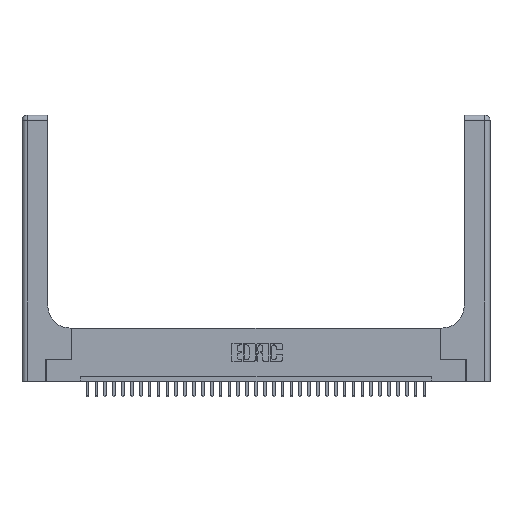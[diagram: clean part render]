
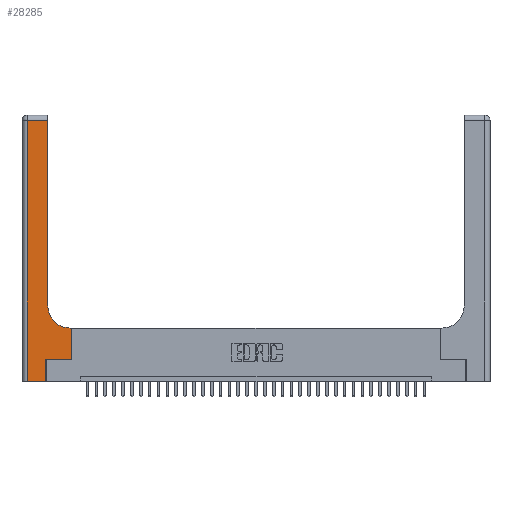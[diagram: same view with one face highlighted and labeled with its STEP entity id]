
A CAD part, top view. The second image highlights one B-rep face of the part: STEP entity #28285.
In plain terms, the highlighted planar face has unit normal (0, 0, 1).
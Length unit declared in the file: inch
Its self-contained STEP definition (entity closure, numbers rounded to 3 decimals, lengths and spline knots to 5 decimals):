
#1178 = VECTOR ( 'NONE', #3255, 39.37008 ) ;
#1307 = CARTESIAN_POINT ( 'NONE',  ( 0.5585, 0.25, 0.37 ) ) ;
#2201 = ORIENTED_EDGE ( 'NONE', *, *, #11558, .T. ) ;
#2996 = EDGE_CURVE ( 'NONE', #31588, #19312, #20535, .T. ) ;
#3020 = VECTOR ( 'NONE', #25640, 39.37008 ) ;
#3255 = DIRECTION ( 'NONE',  ( 1., 0., 0. ) ) ;
#4269 = EDGE_CURVE ( 'NONE', #11643, #11812, #22198, .T. ) ;
#5074 = VECTOR ( 'NONE', #6467, 39.37008 ) ;
#5127 = ORIENTED_EDGE ( 'NONE', *, *, #5555, .T. ) ;
#5555 = EDGE_CURVE ( 'NONE', #18570, #15958, #13162, .T. ) ;
#5947 = LINE ( 'NONE', #6665, #11494 ) ;
#6033 = VECTOR ( 'NONE', #21451, 39.37008 ) ;
#6036 = VECTOR ( 'NONE', #6539, 39.37008 ) ;
#6314 = CARTESIAN_POINT ( 'NONE',  ( 0.5415, 0.85, 0.37 ) ) ;
#6366 = CARTESIAN_POINT ( 'NONE',  ( 0.5585, 0.6, 0.37 ) ) ;
#6467 = DIRECTION ( 'NONE',  ( -1., 0., 0. ) ) ;
#6539 = DIRECTION ( 'NONE',  ( -1., 0., 0. ) ) ;
#6665 = CARTESIAN_POINT ( 'NONE',  ( 0.06, 3., 0.37 ) ) ;
#6705 = EDGE_CURVE ( 'NONE', #7955, #31588, #23958, .T. ) ;
#7124 = CARTESIAN_POINT ( 'NONE',  ( 0.06, 2.94, 0.37 ) ) ;
#7955 = VERTEX_POINT ( 'NONE', #1307 ) ;
#8741 = EDGE_CURVE ( 'NONE', #15958, #8904, #22519, .T. ) ;
#8845 = CARTESIAN_POINT ( 'NONE',  ( 0.269, 0.25, 0.37 ) ) ;
#8904 = VERTEX_POINT ( 'NONE', #7124 ) ;
#11070 = ORIENTED_EDGE ( 'NONE', *, *, #2996, .T. ) ;
#11457 = DIRECTION ( 'NONE',  ( -1., 0., 0. ) ) ;
#11494 = VECTOR ( 'NONE', #26173, 39.37008 ) ;
#11558 = EDGE_CURVE ( 'NONE', #19312, #18570, #18486, .T. ) ;
#11643 = VERTEX_POINT ( 'NONE', #25373 ) ;
#11812 = VERTEX_POINT ( 'NONE', #23815 ) ;
#12047 = AXIS2_PLACEMENT_3D ( 'NONE', #6314, #22192, #25255 ) ;
#12200 = CARTESIAN_POINT ( 'NONE',  ( 0.269, 0., 0.37 ) ) ;
#12456 = LINE ( 'NONE', #12200, #31125 ) ;
#12538 = CARTESIAN_POINT ( 'NONE',  ( 0.5415, 0.6, 0.37 ) ) ;
#13162 = LINE ( 'NONE', #13307, #25482 ) ;
#13307 = CARTESIAN_POINT ( 'NONE',  ( 0.2915, 3., 0.37 ) ) ;
#14546 = EDGE_CURVE ( 'NONE', #11812, #27442, #12456, .T. ) ;
#15958 = VERTEX_POINT ( 'NONE', #30939 ) ;
#16270 = CARTESIAN_POINT ( 'NONE',  ( 0.5585, 0.25, 0.37 ) ) ;
#17266 = CARTESIAN_POINT ( 'NONE',  ( 0., 3., 0.37 ) ) ;
#18011 = EDGE_LOOP ( 'NONE', ( #5127, #34514, #21350, #26608, #22050, #22721, #21574, #11070, #2201 ) ) ;
#18486 = CIRCLE ( 'NONE', #12047, 0.25 ) ;
#18570 = VERTEX_POINT ( 'NONE', #30017 ) ;
#18584 = CARTESIAN_POINT ( 'NONE',  ( 0.269, 0.25, 0.37 ) ) ;
#19312 = VERTEX_POINT ( 'NONE', #12538 ) ;
#19875 = FACE_OUTER_BOUND ( 'NONE', #18011, .T. ) ;
#20535 = LINE ( 'NONE', #33452, #6036 ) ;
#21350 = ORIENTED_EDGE ( 'NONE', *, *, #33008, .T. ) ;
#21451 = DIRECTION ( 'NONE',  ( 0., 1., 0. ) ) ;
#21574 = ORIENTED_EDGE ( 'NONE', *, *, #6705, .T. ) ;
#22050 = ORIENTED_EDGE ( 'NONE', *, *, #14546, .T. ) ;
#22192 = DIRECTION ( 'NONE',  ( 0., 0., -1. ) ) ;
#22198 = LINE ( 'NONE', #22929, #3020 ) ;
#22309 = PLANE ( 'NONE',  #30002 ) ;
#22519 = LINE ( 'NONE', #25758, #5074 ) ;
#22721 = ORIENTED_EDGE ( 'NONE', *, *, #23812, .T. ) ;
#22929 = CARTESIAN_POINT ( 'NONE',  ( 0., 0., 0.37 ) ) ;
#23812 = EDGE_CURVE ( 'NONE', #27442, #7955, #34243, .T. ) ;
#23815 = CARTESIAN_POINT ( 'NONE',  ( 0.269, 0., 0.37 ) ) ;
#23958 = LINE ( 'NONE', #16270, #6033 ) ;
#24001 = DIRECTION ( 'NONE',  ( 0., 1., 0. ) ) ;
#25255 = DIRECTION ( 'NONE',  ( 1., 0., 0. ) ) ;
#25373 = CARTESIAN_POINT ( 'NONE',  ( 0.06, 0., 0.37 ) ) ;
#25482 = VECTOR ( 'NONE', #24001, 39.37008 ) ;
#25640 = DIRECTION ( 'NONE',  ( 1., 0., 0. ) ) ;
#25758 = CARTESIAN_POINT ( 'NONE',  ( 0., 2.94, 0.37 ) ) ;
#26173 = DIRECTION ( 'NONE',  ( 0., -1., 0. ) ) ;
#26608 = ORIENTED_EDGE ( 'NONE', *, *, #4269, .T. ) ;
#27442 = VERTEX_POINT ( 'NONE', #18584 ) ;
#28285 = ADVANCED_FACE ( 'NONE', ( #19875 ), #22309, .F. ) ;
#28328 = DIRECTION ( 'NONE',  ( 0., 1., 0. ) ) ;
#30002 = AXIS2_PLACEMENT_3D ( 'NONE', #17266, #33106, #11457 ) ;
#30017 = CARTESIAN_POINT ( 'NONE',  ( 0.2915, 0.85, 0.37 ) ) ;
#30939 = CARTESIAN_POINT ( 'NONE',  ( 0.2915, 2.94, 0.37 ) ) ;
#31125 = VECTOR ( 'NONE', #28328, 39.37008 ) ;
#31588 = VERTEX_POINT ( 'NONE', #6366 ) ;
#33008 = EDGE_CURVE ( 'NONE', #8904, #11643, #5947, .T. ) ;
#33106 = DIRECTION ( 'NONE',  ( 0., 0., -1. ) ) ;
#33452 = CARTESIAN_POINT ( 'NONE',  ( 0.2915, 0.6, 0.37 ) ) ;
#34243 = LINE ( 'NONE', #8845, #1178 ) ;
#34514 = ORIENTED_EDGE ( 'NONE', *, *, #8741, .T. ) ;
